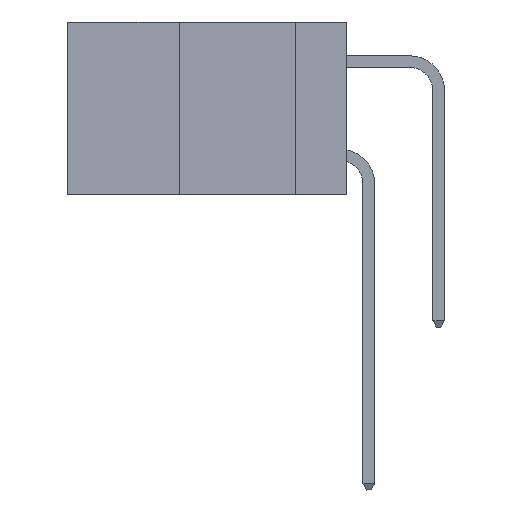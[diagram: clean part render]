
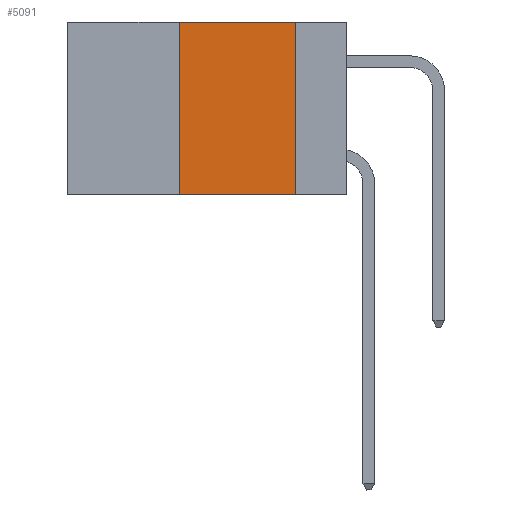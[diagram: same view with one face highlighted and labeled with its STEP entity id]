
A CAD part, left-side view. The second image highlights one B-rep face of the part: STEP entity #5091.
In plain terms, the highlighted planar face has unit normal (-1, 0, 0).
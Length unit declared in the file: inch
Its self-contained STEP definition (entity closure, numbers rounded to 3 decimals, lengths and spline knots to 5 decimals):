
#117 = VERTEX_POINT ( 'NONE', #6600 ) ;
#501 = CARTESIAN_POINT ( 'NONE',  ( 0., 0.36, 0. ) ) ;
#743 = CARTESIAN_POINT ( 'NONE',  ( 0., 0.11, 0. ) ) ;
#2332 = LINE ( 'NONE', #16216, #36537 ) ;
#3371 = DIRECTION ( 'NONE',  ( 0., 0., -1. ) ) ;
#3752 = ORIENTED_EDGE ( 'NONE', *, *, #35468, .F. ) ;
#5091 = ADVANCED_FACE ( 'NONE', ( #5968 ), #20308, .F. ) ;
#5968 = FACE_OUTER_BOUND ( 'NONE', #6988, .T. ) ;
#6090 = CARTESIAN_POINT ( 'NONE',  ( 0., 0.36, 0. ) ) ;
#6318 = LINE ( 'NONE', #20059, #27841 ) ;
#6600 = CARTESIAN_POINT ( 'NONE',  ( 0., 0.11, -0.37 ) ) ;
#6988 = EDGE_LOOP ( 'NONE', ( #32001, #27322, #3752, #38727 ) ) ;
#9097 = EDGE_CURVE ( 'NONE', #10276, #27221, #2332, .T. ) ;
#9615 = CARTESIAN_POINT ( 'NONE',  ( 0., 0.6, 0. ) ) ;
#10276 = VERTEX_POINT ( 'NONE', #6090 ) ;
#10290 = DIRECTION ( 'NONE',  ( 0., 0., -1. ) ) ;
#11512 = EDGE_CURVE ( 'NONE', #27221, #117, #6318, .T. ) ;
#15254 = VECTOR ( 'NONE', #34650, 39.37008 ) ;
#16216 = CARTESIAN_POINT ( 'NONE',  ( 0., 0.6, 0. ) ) ;
#17376 = LINE ( 'NONE', #501, #35902 ) ;
#18084 = VERTEX_POINT ( 'NONE', #38985 ) ;
#19686 = EDGE_CURVE ( 'NONE', #18084, #117, #20982, .T. ) ;
#20059 = CARTESIAN_POINT ( 'NONE',  ( 0., 0.11, 0. ) ) ;
#20308 = PLANE ( 'NONE',  #39170 ) ;
#20982 = LINE ( 'NONE', #24621, #15254 ) ;
#24621 = CARTESIAN_POINT ( 'NONE',  ( 0., 0.6, -0.37 ) ) ;
#24866 = DIRECTION ( 'NONE',  ( 0., 0., 1. ) ) ;
#26019 = DIRECTION ( 'NONE',  ( 0., -1., 0. ) ) ;
#27221 = VERTEX_POINT ( 'NONE', #743 ) ;
#27322 = ORIENTED_EDGE ( 'NONE', *, *, #9097, .F. ) ;
#27841 = VECTOR ( 'NONE', #3371, 39.37008 ) ;
#32001 = ORIENTED_EDGE ( 'NONE', *, *, #11512, .F. ) ;
#34422 = DIRECTION ( 'NONE',  ( 1., 0., 0. ) ) ;
#34650 = DIRECTION ( 'NONE',  ( 0., -1., 0. ) ) ;
#35468 = EDGE_CURVE ( 'NONE', #18084, #10276, #17376, .T. ) ;
#35902 = VECTOR ( 'NONE', #24866, 39.37008 ) ;
#36537 = VECTOR ( 'NONE', #26019, 39.37008 ) ;
#38727 = ORIENTED_EDGE ( 'NONE', *, *, #19686, .T. ) ;
#38985 = CARTESIAN_POINT ( 'NONE',  ( 0., 0.36, -0.37 ) ) ;
#39170 = AXIS2_PLACEMENT_3D ( 'NONE', #9615, #34422, #10290 ) ;
